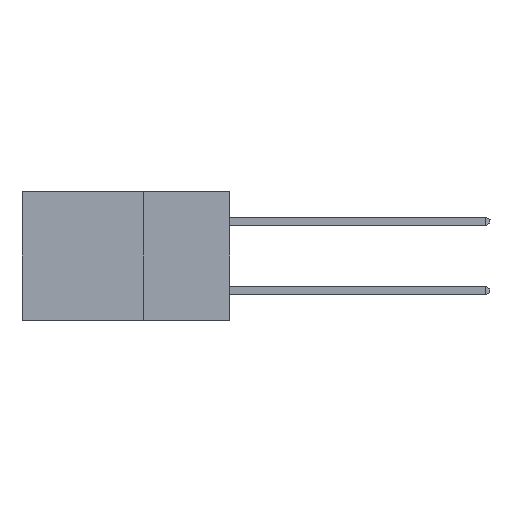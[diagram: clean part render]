
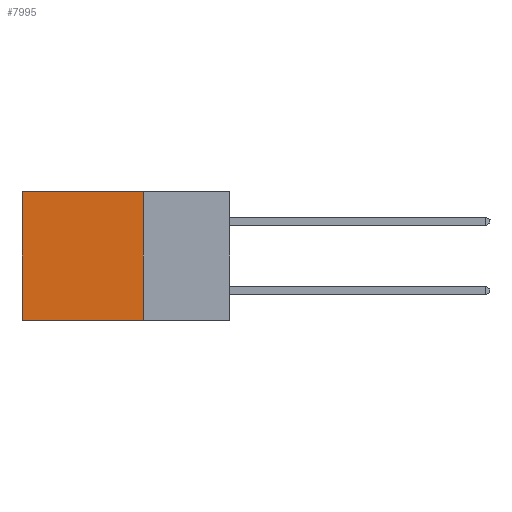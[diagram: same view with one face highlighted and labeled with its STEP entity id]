
A CAD part, left-side view. The second image highlights one B-rep face of the part: STEP entity #7995.
In plain terms, the highlighted planar face has unit normal (-1, 0, 0).
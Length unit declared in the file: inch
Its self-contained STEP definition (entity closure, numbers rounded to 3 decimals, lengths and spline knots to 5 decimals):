
#115 = EDGE_LOOP ( 'NONE', ( #5620, #5211, #5051, #13823 ) ) ;
#334 = VECTOR ( 'NONE', #1401, 39.37008 ) ;
#346 = FACE_OUTER_BOUND ( 'NONE', #115, .T. ) ;
#411 = DIRECTION ( 'NONE',  ( 0., 0., -1. ) ) ;
#1094 = AXIS2_PLACEMENT_3D ( 'NONE', #3231, #1135, #3419 ) ;
#1135 = DIRECTION ( 'NONE',  ( 1., 0., 0. ) ) ;
#1348 = CARTESIAN_POINT ( 'NONE',  ( 0.298, 0.6, -0.37 ) ) ;
#1401 = DIRECTION ( 'NONE',  ( 0., 1., 0. ) ) ;
#1817 = CARTESIAN_POINT ( 'NONE',  ( 0.298, 0.25, 0. ) ) ;
#2205 = VECTOR ( 'NONE', #10025, 39.37008 ) ;
#2802 = VECTOR ( 'NONE', #411, 39.37008 ) ;
#3231 = CARTESIAN_POINT ( 'NONE',  ( 0.298, 0.25, 0. ) ) ;
#3419 = DIRECTION ( 'NONE',  ( 0., 0., -1. ) ) ;
#3848 = LINE ( 'NONE', #5762, #2205 ) ;
#4418 = CARTESIAN_POINT ( 'NONE',  ( 0.298, 0.25, 0. ) ) ;
#4771 = VERTEX_POINT ( 'NONE', #4418 ) ;
#5051 = ORIENTED_EDGE ( 'NONE', *, *, #10023, .F. ) ;
#5211 = ORIENTED_EDGE ( 'NONE', *, *, #6421, .F. ) ;
#5620 = ORIENTED_EDGE ( 'NONE', *, *, #11060, .T. ) ;
#5762 = CARTESIAN_POINT ( 'NONE',  ( 0.298, 0.25, -0.37 ) ) ;
#6421 = EDGE_CURVE ( 'NONE', #10149, #6432, #3848, .T. ) ;
#6432 = VERTEX_POINT ( 'NONE', #1348 ) ;
#6851 = CARTESIAN_POINT ( 'NONE',  ( 0.298, 0.6, 0. ) ) ;
#7371 = EDGE_CURVE ( 'NONE', #4771, #11751, #9538, .T. ) ;
#7995 = ADVANCED_FACE ( 'NONE', ( #346 ), #11968, .F. ) ;
#8515 = LINE ( 'NONE', #6851, #2802 ) ;
#8547 = LINE ( 'NONE', #1817, #13227 ) ;
#9538 = LINE ( 'NONE', #10908, #334 ) ;
#10023 = EDGE_CURVE ( 'NONE', #4771, #10149, #8547, .T. ) ;
#10025 = DIRECTION ( 'NONE',  ( 0., 1., 0. ) ) ;
#10149 = VERTEX_POINT ( 'NONE', #13247 ) ;
#10908 = CARTESIAN_POINT ( 'NONE',  ( 0.298, 0.25, 0. ) ) ;
#11060 = EDGE_CURVE ( 'NONE', #11751, #6432, #8515, .T. ) ;
#11751 = VERTEX_POINT ( 'NONE', #13764 ) ;
#11968 = PLANE ( 'NONE',  #1094 ) ;
#13227 = VECTOR ( 'NONE', #13660, 39.37008 ) ;
#13247 = CARTESIAN_POINT ( 'NONE',  ( 0.298, 0.25, -0.37 ) ) ;
#13660 = DIRECTION ( 'NONE',  ( 0., 0., -1. ) ) ;
#13764 = CARTESIAN_POINT ( 'NONE',  ( 0.298, 0.6, 0. ) ) ;
#13823 = ORIENTED_EDGE ( 'NONE', *, *, #7371, .T. ) ;
